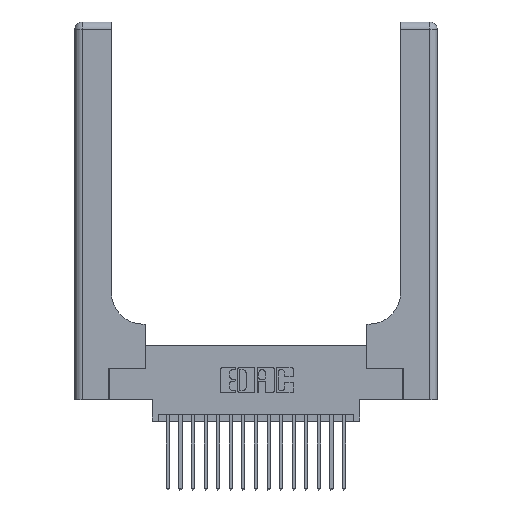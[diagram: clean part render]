
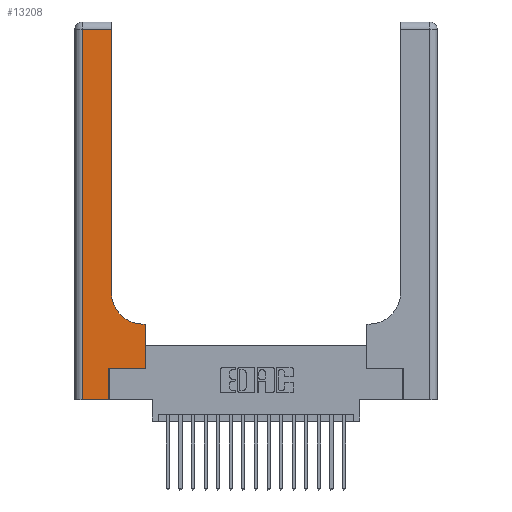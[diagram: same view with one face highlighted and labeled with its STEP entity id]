
A CAD part, top view. The second image highlights one B-rep face of the part: STEP entity #13208.
In plain terms, the highlighted planar face has unit normal (0, 0, 1).
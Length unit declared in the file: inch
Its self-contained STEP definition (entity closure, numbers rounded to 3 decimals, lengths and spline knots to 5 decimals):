
#401 = DIRECTION ( 'NONE',  ( -1., 0., 0. ) ) ;
#670 = VERTEX_POINT ( 'NONE', #19833 ) ;
#1814 = CARTESIAN_POINT ( 'NONE',  ( 0.5585, 0.6, 0.37 ) ) ;
#1875 = VECTOR ( 'NONE', #4896, 39.37008 ) ;
#2159 = VERTEX_POINT ( 'NONE', #4852 ) ;
#2413 = LINE ( 'NONE', #4158, #10000 ) ;
#2582 = ORIENTED_EDGE ( 'NONE', *, *, #9530, .T. ) ;
#2831 = AXIS2_PLACEMENT_3D ( 'NONE', #13842, #16839, #17048 ) ;
#2863 = LINE ( 'NONE', #9449, #15951 ) ;
#2898 = DIRECTION ( 'NONE',  ( 0., 1., 0. ) ) ;
#3289 = VERTEX_POINT ( 'NONE', #11303 ) ;
#4158 = CARTESIAN_POINT ( 'NONE',  ( 0.06, 3., 0.37 ) ) ;
#4219 = PLANE ( 'NONE',  #2831 ) ;
#4305 = VERTEX_POINT ( 'NONE', #11195 ) ;
#4454 = DIRECTION ( 'NONE',  ( 1., 0., 0. ) ) ;
#4577 = DIRECTION ( 'NONE',  ( 0., 1., 0. ) ) ;
#4852 = CARTESIAN_POINT ( 'NONE',  ( 0.5415, 0.6, 0.37 ) ) ;
#4896 = DIRECTION ( 'NONE',  ( 0., 1., 0. ) ) ;
#5215 = ORIENTED_EDGE ( 'NONE', *, *, #6471, .T. ) ;
#5447 = EDGE_CURVE ( 'NONE', #15061, #2159, #14999, .T. ) ;
#5547 = CARTESIAN_POINT ( 'NONE',  ( 0.2915, 0.85, 0.37 ) ) ;
#6102 = CARTESIAN_POINT ( 'NONE',  ( 0.5415, 0.85, 0.37 ) ) ;
#6197 = LINE ( 'NONE', #11484, #1875 ) ;
#6307 = CARTESIAN_POINT ( 'NONE',  ( 0.2915, 3., 0.37 ) ) ;
#6471 = EDGE_CURVE ( 'NONE', #670, #11350, #2863, .T. ) ;
#6607 = ORIENTED_EDGE ( 'NONE', *, *, #12854, .T. ) ;
#7812 = CARTESIAN_POINT ( 'NONE',  ( 0.06, 0., 0.37 ) ) ;
#8014 = EDGE_CURVE ( 'NONE', #17896, #3289, #14644, .T. ) ;
#8126 = ORIENTED_EDGE ( 'NONE', *, *, #12221, .T. ) ;
#8159 = ORIENTED_EDGE ( 'NONE', *, *, #14525, .T. ) ;
#8609 = VECTOR ( 'NONE', #2898, 39.37008 ) ;
#9308 = VECTOR ( 'NONE', #20211, 39.37008 ) ;
#9449 = CARTESIAN_POINT ( 'NONE',  ( 0.269, 0., 0.37 ) ) ;
#9530 = EDGE_CURVE ( 'NONE', #11350, #4305, #18794, .T. ) ;
#10000 = VECTOR ( 'NONE', #11946, 39.37008 ) ;
#10266 = CARTESIAN_POINT ( 'NONE',  ( 0., 2.94, 0.37 ) ) ;
#11151 = CARTESIAN_POINT ( 'NONE',  ( 0.269, 0.25, 0.37 ) ) ;
#11195 = CARTESIAN_POINT ( 'NONE',  ( 0.5585, 0.25, 0.37 ) ) ;
#11239 = DIRECTION ( 'NONE',  ( 1., 0., 0. ) ) ;
#11303 = CARTESIAN_POINT ( 'NONE',  ( 0.2915, 2.94, 0.37 ) ) ;
#11350 = VERTEX_POINT ( 'NONE', #11151 ) ;
#11442 = CARTESIAN_POINT ( 'NONE',  ( 0., 0., 0.37 ) ) ;
#11462 = EDGE_CURVE ( 'NONE', #13882, #18157, #2413, .T. ) ;
#11484 = CARTESIAN_POINT ( 'NONE',  ( 0.5585, 0.25, 0.37 ) ) ;
#11946 = DIRECTION ( 'NONE',  ( 0., -1., 0. ) ) ;
#12221 = EDGE_CURVE ( 'NONE', #18157, #670, #17945, .T. ) ;
#12779 = ORIENTED_EDGE ( 'NONE', *, *, #5447, .T. ) ;
#12854 = EDGE_CURVE ( 'NONE', #4305, #15061, #6197, .T. ) ;
#13208 = ADVANCED_FACE ( 'NONE', ( #20691 ), #4219, .F. ) ;
#13567 = EDGE_LOOP ( 'NONE', ( #19414, #19395, #19657, #8126, #5215, #2582, #6607, #12779, #8159 ) ) ;
#13842 = CARTESIAN_POINT ( 'NONE',  ( 0., 3., 0.37 ) ) ;
#13882 = VERTEX_POINT ( 'NONE', #17159 ) ;
#14525 = EDGE_CURVE ( 'NONE', #2159, #17896, #18620, .T. ) ;
#14644 = LINE ( 'NONE', #6307, #8609 ) ;
#14980 = VECTOR ( 'NONE', #11239, 39.37008 ) ;
#14999 = LINE ( 'NONE', #16658, #15987 ) ;
#15061 = VERTEX_POINT ( 'NONE', #1814 ) ;
#15150 = DIRECTION ( 'NONE',  ( -1., 0., 0. ) ) ;
#15951 = VECTOR ( 'NONE', #4577, 39.37008 ) ;
#15987 = VECTOR ( 'NONE', #401, 39.37008 ) ;
#16405 = EDGE_CURVE ( 'NONE', #3289, #13882, #16435, .T. ) ;
#16435 = LINE ( 'NONE', #10266, #18153 ) ;
#16658 = CARTESIAN_POINT ( 'NONE',  ( 0.2915, 0.6, 0.37 ) ) ;
#16839 = DIRECTION ( 'NONE',  ( 0., 0., -1. ) ) ;
#17048 = DIRECTION ( 'NONE',  ( -1., 0., 0. ) ) ;
#17159 = CARTESIAN_POINT ( 'NONE',  ( 0.06, 2.94, 0.37 ) ) ;
#17333 = DIRECTION ( 'NONE',  ( 0., 0., -1. ) ) ;
#17896 = VERTEX_POINT ( 'NONE', #5547 ) ;
#17945 = LINE ( 'NONE', #11442, #14980 ) ;
#18153 = VECTOR ( 'NONE', #15150, 39.37008 ) ;
#18157 = VERTEX_POINT ( 'NONE', #7812 ) ;
#18620 = CIRCLE ( 'NONE', #19103, 0.25 ) ;
#18794 = LINE ( 'NONE', #18812, #9308 ) ;
#18812 = CARTESIAN_POINT ( 'NONE',  ( 0.269, 0.25, 0.37 ) ) ;
#19103 = AXIS2_PLACEMENT_3D ( 'NONE', #6102, #17333, #4454 ) ;
#19395 = ORIENTED_EDGE ( 'NONE', *, *, #16405, .T. ) ;
#19414 = ORIENTED_EDGE ( 'NONE', *, *, #8014, .T. ) ;
#19657 = ORIENTED_EDGE ( 'NONE', *, *, #11462, .T. ) ;
#19833 = CARTESIAN_POINT ( 'NONE',  ( 0.269, 0., 0.37 ) ) ;
#20211 = DIRECTION ( 'NONE',  ( 1., 0., 0. ) ) ;
#20691 = FACE_OUTER_BOUND ( 'NONE', #13567, .T. ) ;
